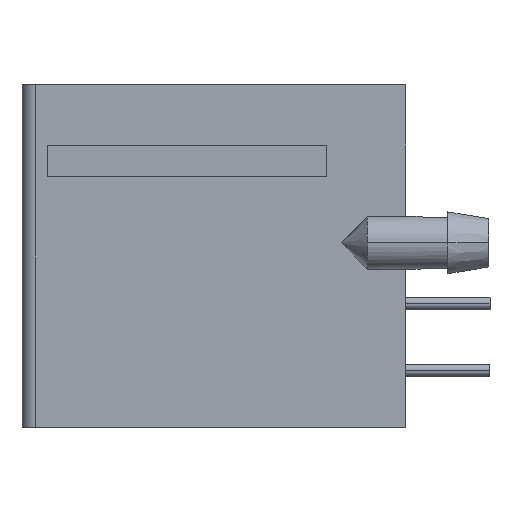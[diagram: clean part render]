
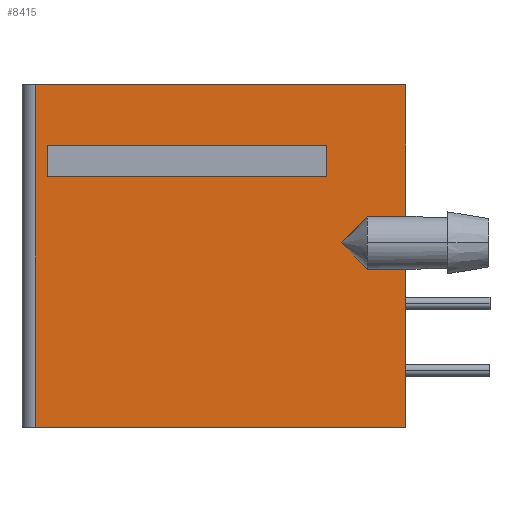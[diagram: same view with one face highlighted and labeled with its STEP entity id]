
A CAD part, left-side view. The second image highlights one B-rep face of the part: STEP entity #8415.
In plain terms, the highlighted planar face has unit normal (-1, 0, 0).
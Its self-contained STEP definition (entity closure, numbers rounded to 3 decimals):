
#63 = CARTESIAN_POINT ( 'NONE',  ( -11.65, -0.281, 10.7 ) ) ;
#729 = VERTEX_POINT ( 'NONE', #16103 ) ;
#843 = VERTEX_POINT ( 'NONE', #8854 ) ;
#1293 = DIRECTION ( 'NONE',  ( -1., 0., 0. ) ) ;
#1302 = EDGE_CURVE ( 'NONE', #13822, #17679, #6335, .T. ) ;
#1479 = LINE ( 'NONE', #5333, #1905 ) ;
#1482 = EDGE_CURVE ( 'NONE', #12422, #3798, #11125, .T. ) ;
#1905 = VECTOR ( 'NONE', #14004, 1000. ) ;
#1941 = VECTOR ( 'NONE', #16805, 1000. ) ;
#2001 = EDGE_CURVE ( 'NONE', #10660, #17966, #10672, .T. ) ;
#2082 = CARTESIAN_POINT ( 'NONE',  ( -11.65, 0., 13. ) ) ;
#2281 = CARTESIAN_POINT ( 'NONE',  ( -11.65, 2.45, 7. ) ) ;
#2462 = DIRECTION ( 'NONE',  ( 0., -0.707, 0.707 ) ) ;
#2575 = CARTESIAN_POINT ( 'NONE',  ( -11.65, -0.281, 9.5 ) ) ;
#2735 = LINE ( 'NONE', #15197, #9071 ) ;
#2815 = CARTESIAN_POINT ( 'NONE',  ( -11.65, 2.45, 7. ) ) ;
#3160 = EDGE_CURVE ( 'NONE', #17966, #18047, #8852, .T. ) ;
#3243 = ORIENTED_EDGE ( 'NONE', *, *, #6000, .T. ) ;
#3248 = EDGE_CURVE ( 'NONE', #9276, #729, #4295, .T. ) ;
#3251 = ORIENTED_EDGE ( 'NONE', *, *, #1482, .F. ) ;
#3416 = VERTEX_POINT ( 'NONE', #2082 ) ;
#3451 = FACE_OUTER_BOUND ( 'NONE', #9798, .T. ) ;
#3533 = ORIENTED_EDGE ( 'NONE', *, *, #12097, .F. ) ;
#3683 = EDGE_CURVE ( 'NONE', #12422, #3416, #5137, .T. ) ;
#3798 = VERTEX_POINT ( 'NONE', #12039 ) ;
#3842 = ORIENTED_EDGE ( 'NONE', *, *, #17318, .T. ) ;
#3844 = CARTESIAN_POINT ( 'NONE',  ( -11.65, 1.45, 6. ) ) ;
#4054 = ORIENTED_EDGE ( 'NONE', *, *, #11242, .T. ) ;
#4125 = DIRECTION ( 'NONE',  ( 0., -1., 0. ) ) ;
#4295 = LINE ( 'NONE', #6195, #17448 ) ;
#4644 = LINE ( 'NONE', #4765, #8552 ) ;
#4765 = CARTESIAN_POINT ( 'NONE',  ( -11.65, -0.281, 13. ) ) ;
#4844 = CARTESIAN_POINT ( 'NONE',  ( -11.65, 0., -0.26 ) ) ;
#5009 = CARTESIAN_POINT ( 'NONE',  ( -11.65, 13.6, 10.7 ) ) ;
#5137 = LINE ( 'NONE', #4844, #9052 ) ;
#5333 = CARTESIAN_POINT ( 'NONE',  ( -11.65, 3., -0.26 ) ) ;
#5502 = LINE ( 'NONE', #63, #10719 ) ;
#5672 = CARTESIAN_POINT ( 'NONE',  ( -11.65, 14.05, 13. ) ) ;
#5816 = CARTESIAN_POINT ( 'NONE',  ( -11.65, 0., 0. ) ) ;
#6000 = EDGE_CURVE ( 'NONE', #17800, #6657, #11593, .T. ) ;
#6083 = ORIENTED_EDGE ( 'NONE', *, *, #3248, .T. ) ;
#6116 = VECTOR ( 'NONE', #6643, 1000. ) ;
#6195 = CARTESIAN_POINT ( 'NONE',  ( -11.65, 14.05, -0.26 ) ) ;
#6335 = LINE ( 'NONE', #3844, #6116 ) ;
#6524 = ORIENTED_EDGE ( 'NONE', *, *, #2001, .T. ) ;
#6561 = CARTESIAN_POINT ( 'NONE',  ( -11.65, 0., 8. ) ) ;
#6643 = DIRECTION ( 'NONE',  ( 0., 0.707, 0.707 ) ) ;
#6657 = VERTEX_POINT ( 'NONE', #17206 ) ;
#6806 = DIRECTION ( 'NONE',  ( 0., 1., 0. ) ) ;
#6815 = DIRECTION ( 'NONE',  ( 0., -1., 0. ) ) ;
#6993 = CARTESIAN_POINT ( 'NONE',  ( -11.65, 0., 8. ) ) ;
#7044 = PLANE ( 'NONE',  #16260 ) ;
#7178 = ORIENTED_EDGE ( 'NONE', *, *, #1302, .T. ) ;
#7411 = DIRECTION ( 'NONE',  ( 0., 0., -1. ) ) ;
#7621 = DIRECTION ( 'NONE',  ( 0., 1., 0. ) ) ;
#8058 = VECTOR ( 'NONE', #6806, 1000. ) ;
#8237 = FACE_BOUND ( 'NONE', #10113, .T. ) ;
#8415 = ADVANCED_FACE ( 'NONE', ( #3451, #8237 ), #7044, .T. ) ;
#8552 = VECTOR ( 'NONE', #7621, 1000. ) ;
#8852 = LINE ( 'NONE', #17116, #9070 ) ;
#8854 = CARTESIAN_POINT ( 'NONE',  ( -11.65, 3., 10.7 ) ) ;
#8916 = EDGE_CURVE ( 'NONE', #3416, #9276, #4644, .T. ) ;
#9005 = CARTESIAN_POINT ( 'NONE',  ( -11.65, 0., -0.26 ) ) ;
#9052 = VECTOR ( 'NONE', #14621, 1000. ) ;
#9070 = VECTOR ( 'NONE', #13146, 1000. ) ;
#9071 = VECTOR ( 'NONE', #6815, 1000. ) ;
#9276 = VERTEX_POINT ( 'NONE', #5672 ) ;
#9619 = CARTESIAN_POINT ( 'NONE',  ( -11.65, 1.45, 6. ) ) ;
#9798 = EDGE_LOOP ( 'NONE', ( #6083, #16212, #3243, #3533, #7178, #18079, #3251, #17828, #13153 ) ) ;
#10113 = EDGE_LOOP ( 'NONE', ( #16022, #3842, #4054, #6524 ) ) ;
#10416 = DIRECTION ( 'NONE',  ( 0., 0., 1. ) ) ;
#10605 = CARTESIAN_POINT ( 'NONE',  ( -11.65, -0.281, 0. ) ) ;
#10660 = VERTEX_POINT ( 'NONE', #10718 ) ;
#10672 = LINE ( 'NONE', #2575, #8058 ) ;
#10718 = CARTESIAN_POINT ( 'NONE',  ( -11.65, 3., 9.5 ) ) ;
#10719 = VECTOR ( 'NONE', #16980, 1000. ) ;
#11125 = LINE ( 'NONE', #6993, #1941 ) ;
#11242 = EDGE_CURVE ( 'NONE', #843, #10660, #1479, .T. ) ;
#11593 = LINE ( 'NONE', #9005, #13120 ) ;
#11601 = CARTESIAN_POINT ( 'NONE',  ( -11.65, 13.6, 9.5 ) ) ;
#11936 = EDGE_CURVE ( 'NONE', #17679, #3798, #16118, .T. ) ;
#12039 = CARTESIAN_POINT ( 'NONE',  ( -11.65, 1.45, 8. ) ) ;
#12097 = EDGE_CURVE ( 'NONE', #13822, #6657, #2735, .T. ) ;
#12422 = VERTEX_POINT ( 'NONE', #6561 ) ;
#13120 = VECTOR ( 'NONE', #10416, 1000. ) ;
#13146 = DIRECTION ( 'NONE',  ( 0., 0., 1. ) ) ;
#13153 = ORIENTED_EDGE ( 'NONE', *, *, #8916, .T. ) ;
#13458 = VECTOR ( 'NONE', #2462, 1000. ) ;
#13822 = VERTEX_POINT ( 'NONE', #9619 ) ;
#14004 = DIRECTION ( 'NONE',  ( 0., 0., -1. ) ) ;
#14621 = DIRECTION ( 'NONE',  ( 0., 0., 1. ) ) ;
#15197 = CARTESIAN_POINT ( 'NONE',  ( -11.65, 0., 6. ) ) ;
#15255 = CARTESIAN_POINT ( 'NONE',  ( -11.65, -0.281, -0.26 ) ) ;
#15311 = EDGE_CURVE ( 'NONE', #729, #17800, #17840, .T. ) ;
#16022 = ORIENTED_EDGE ( 'NONE', *, *, #3160, .T. ) ;
#16103 = CARTESIAN_POINT ( 'NONE',  ( -11.65, 14.05, 0. ) ) ;
#16118 = LINE ( 'NONE', #2281, #13458 ) ;
#16212 = ORIENTED_EDGE ( 'NONE', *, *, #15311, .T. ) ;
#16260 = AXIS2_PLACEMENT_3D ( 'NONE', #15255, #1293, #4125 ) ;
#16279 = VECTOR ( 'NONE', #17832, 1000. ) ;
#16805 = DIRECTION ( 'NONE',  ( 0., 1., 0. ) ) ;
#16980 = DIRECTION ( 'NONE',  ( 0., -1., 0. ) ) ;
#17116 = CARTESIAN_POINT ( 'NONE',  ( -11.65, 13.6, -0.26 ) ) ;
#17206 = CARTESIAN_POINT ( 'NONE',  ( -11.65, 0., 6. ) ) ;
#17318 = EDGE_CURVE ( 'NONE', #18047, #843, #5502, .T. ) ;
#17448 = VECTOR ( 'NONE', #7411, 1000. ) ;
#17679 = VERTEX_POINT ( 'NONE', #2815 ) ;
#17800 = VERTEX_POINT ( 'NONE', #5816 ) ;
#17828 = ORIENTED_EDGE ( 'NONE', *, *, #3683, .T. ) ;
#17832 = DIRECTION ( 'NONE',  ( 0., -1., 0. ) ) ;
#17840 = LINE ( 'NONE', #10605, #16279 ) ;
#17966 = VERTEX_POINT ( 'NONE', #11601 ) ;
#18047 = VERTEX_POINT ( 'NONE', #5009 ) ;
#18079 = ORIENTED_EDGE ( 'NONE', *, *, #11936, .T. ) ;
